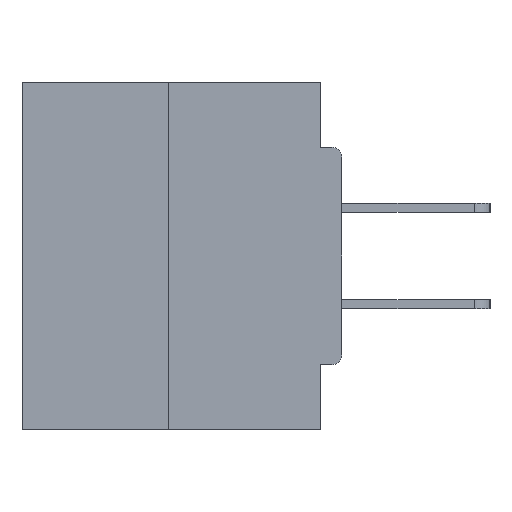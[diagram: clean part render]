
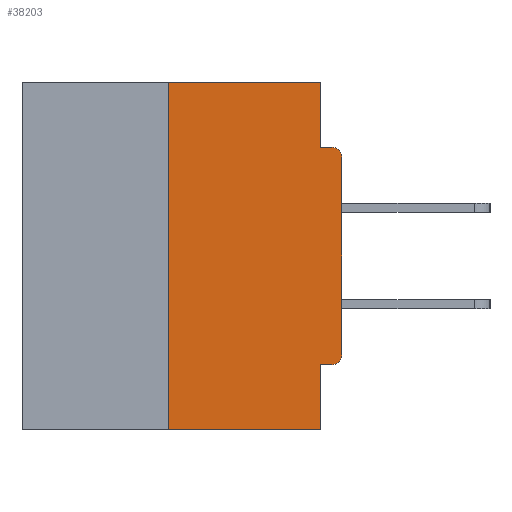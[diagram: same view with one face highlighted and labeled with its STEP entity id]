
A CAD part, left-side view. The second image highlights one B-rep face of the part: STEP entity #38203.
In plain terms, the highlighted planar face has unit normal (-1, 0, 0).
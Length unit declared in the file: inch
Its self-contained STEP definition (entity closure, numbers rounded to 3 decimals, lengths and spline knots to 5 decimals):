
#847 = EDGE_CURVE ( 'NONE', #22182, #23915, #11030, .T. ) ;
#1805 = EDGE_CURVE ( 'NONE', #14706, #38209, #2296, .T. ) ;
#1825 = CARTESIAN_POINT ( 'NONE',  ( 0., 0.031, -0.5 ) ) ;
#2225 = DIRECTION ( 'NONE',  ( 0., 0., -1. ) ) ;
#2296 = LINE ( 'NONE', #13891, #9530 ) ;
#3049 = VERTEX_POINT ( 'NONE', #26535 ) ;
#3992 = CARTESIAN_POINT ( 'NONE',  ( 0., 0.015, -0.3915 ) ) ;
#4007 = DIRECTION ( 'NONE',  ( 0., 1., 0. ) ) ;
#4258 = CARTESIAN_POINT ( 'NONE',  ( 0., 0., -0.4065 ) ) ;
#4341 = FACE_OUTER_BOUND ( 'NONE', #24311, .T. ) ;
#5800 = CARTESIAN_POINT ( 'NONE',  ( 0., 0.031, -0.5 ) ) ;
#5937 = DIRECTION ( 'NONE',  ( 0., 0., -1. ) ) ;
#6276 = CARTESIAN_POINT ( 'NONE',  ( 0., 0.031, -0.4065 ) ) ;
#6288 = ORIENTED_EDGE ( 'NONE', *, *, #16903, .F. ) ;
#6961 = CARTESIAN_POINT ( 'NONE',  ( 0., 0.46, 0. ) ) ;
#7263 = VECTOR ( 'NONE', #2225, 39.37008 ) ;
#7346 = EDGE_CURVE ( 'NONE', #29264, #22182, #22488, .T. ) ;
#8765 = AXIS2_PLACEMENT_3D ( 'NONE', #15200, #14786, #5937 ) ;
#9530 = VECTOR ( 'NONE', #20177, 39.37008 ) ;
#9549 = EDGE_CURVE ( 'NONE', #23915, #3049, #39599, .T. ) ;
#9751 = LINE ( 'NONE', #6961, #35659 ) ;
#9938 = VERTEX_POINT ( 'NONE', #11224 ) ;
#10696 = EDGE_CURVE ( 'NONE', #29264, #37270, #11575, .T. ) ;
#11030 = LINE ( 'NONE', #11891, #37954 ) ;
#11224 = CARTESIAN_POINT ( 'NONE',  ( 0., 0.031, -0.0935 ) ) ;
#11429 = CARTESIAN_POINT ( 'NONE',  ( 0., 0.25, 0. ) ) ;
#11575 = LINE ( 'NONE', #4258, #15914 ) ;
#11625 = ORIENTED_EDGE ( 'NONE', *, *, #7346, .T. ) ;
#11891 = CARTESIAN_POINT ( 'NONE',  ( 0., 0., 0. ) ) ;
#13891 = CARTESIAN_POINT ( 'NONE',  ( 0., 0.46, -0.5 ) ) ;
#14329 = DIRECTION ( 'NONE',  ( 0., 0., 1. ) ) ;
#14706 = VERTEX_POINT ( 'NONE', #37978 ) ;
#14786 = DIRECTION ( 'NONE',  ( 1., 0., 0. ) ) ;
#14925 = DIRECTION ( 'NONE',  ( 0., 0., -1. ) ) ;
#15200 = CARTESIAN_POINT ( 'NONE',  ( 0., 0.46, 0. ) ) ;
#15381 = ORIENTED_EDGE ( 'NONE', *, *, #847, .T. ) ;
#15636 = ORIENTED_EDGE ( 'NONE', *, *, #36289, .F. ) ;
#15914 = VECTOR ( 'NONE', #4007, 39.37008 ) ;
#15955 = DIRECTION ( 'NONE',  ( -1., 0., 0. ) ) ;
#16216 = EDGE_CURVE ( 'NONE', #9938, #3049, #35032, .T. ) ;
#16801 = ORIENTED_EDGE ( 'NONE', *, *, #16216, .F. ) ;
#16903 = EDGE_CURVE ( 'NONE', #20924, #9938, #39352, .T. ) ;
#17598 = EDGE_CURVE ( 'NONE', #14706, #22510, #24403, .T. ) ;
#17629 = AXIS2_PLACEMENT_3D ( 'NONE', #3992, #15955, #18786 ) ;
#17657 = DIRECTION ( 'NONE',  ( 0., 0., -1. ) ) ;
#18786 = DIRECTION ( 'NONE',  ( 0., 0., -1. ) ) ;
#20177 = DIRECTION ( 'NONE',  ( 0., -1., 0. ) ) ;
#20194 = ORIENTED_EDGE ( 'NONE', *, *, #9549, .T. ) ;
#20239 = LINE ( 'NONE', #1825, #7263 ) ;
#20420 = ORIENTED_EDGE ( 'NONE', *, *, #17598, .F. ) ;
#20924 = VERTEX_POINT ( 'NONE', #34156 ) ;
#21965 = ORIENTED_EDGE ( 'NONE', *, *, #1805, .T. ) ;
#22182 = VERTEX_POINT ( 'NONE', #30410 ) ;
#22488 = CIRCLE ( 'NONE', #17629, 0.015 ) ;
#22510 = VERTEX_POINT ( 'NONE', #11429 ) ;
#23476 = VECTOR ( 'NONE', #36313, 39.37008 ) ;
#23889 = PLANE ( 'NONE',  #8765 ) ;
#23915 = VERTEX_POINT ( 'NONE', #32828 ) ;
#24311 = EDGE_LOOP ( 'NONE', ( #15636, #20420, #21965, #29611, #28047, #11625, #15381, #20194, #16801, #6288 ) ) ;
#24403 = LINE ( 'NONE', #26783, #29672 ) ;
#26233 = CARTESIAN_POINT ( 'NONE',  ( 0., 0.015, -0.4065 ) ) ;
#26295 = VECTOR ( 'NONE', #17657, 39.37008 ) ;
#26535 = CARTESIAN_POINT ( 'NONE',  ( 0., 0.015, -0.0935 ) ) ;
#26783 = CARTESIAN_POINT ( 'NONE',  ( 0., 0.25, 0. ) ) ;
#26846 = CARTESIAN_POINT ( 'NONE',  ( 0., 0.015, -0.1085 ) ) ;
#26980 = DIRECTION ( 'NONE',  ( -1., 0., 0. ) ) ;
#28047 = ORIENTED_EDGE ( 'NONE', *, *, #10696, .F. ) ;
#29264 = VERTEX_POINT ( 'NONE', #26233 ) ;
#29611 = ORIENTED_EDGE ( 'NONE', *, *, #37084, .F. ) ;
#29672 = VECTOR ( 'NONE', #14329, 39.37008 ) ;
#30256 = AXIS2_PLACEMENT_3D ( 'NONE', #26846, #26980, #14925 ) ;
#30410 = CARTESIAN_POINT ( 'NONE',  ( 0., 0., -0.3915 ) ) ;
#32828 = CARTESIAN_POINT ( 'NONE',  ( 0., 0., -0.1085 ) ) ;
#34156 = CARTESIAN_POINT ( 'NONE',  ( 0., 0.031, 0. ) ) ;
#34302 = DIRECTION ( 'NONE',  ( 0., 0., 1. ) ) ;
#34904 = DIRECTION ( 'NONE',  ( 0., -1., 0. ) ) ;
#35032 = LINE ( 'NONE', #35904, #23476 ) ;
#35659 = VECTOR ( 'NONE', #34904, 39.37008 ) ;
#35904 = CARTESIAN_POINT ( 'NONE',  ( 0., 0., -0.0935 ) ) ;
#36289 = EDGE_CURVE ( 'NONE', #22510, #20924, #9751, .T. ) ;
#36313 = DIRECTION ( 'NONE',  ( 0., -1., 0. ) ) ;
#37084 = EDGE_CURVE ( 'NONE', #37270, #38209, #20239, .T. ) ;
#37270 = VERTEX_POINT ( 'NONE', #6276 ) ;
#37954 = VECTOR ( 'NONE', #34302, 39.37008 ) ;
#37978 = CARTESIAN_POINT ( 'NONE',  ( 0., 0.25, -0.5 ) ) ;
#38203 = ADVANCED_FACE ( 'NONE', ( #4341 ), #23889, .F. ) ;
#38209 = VERTEX_POINT ( 'NONE', #5800 ) ;
#39008 = CARTESIAN_POINT ( 'NONE',  ( 0., 0.031, 0. ) ) ;
#39352 = LINE ( 'NONE', #39008, #26295 ) ;
#39599 = CIRCLE ( 'NONE', #30256, 0.015 ) ;
